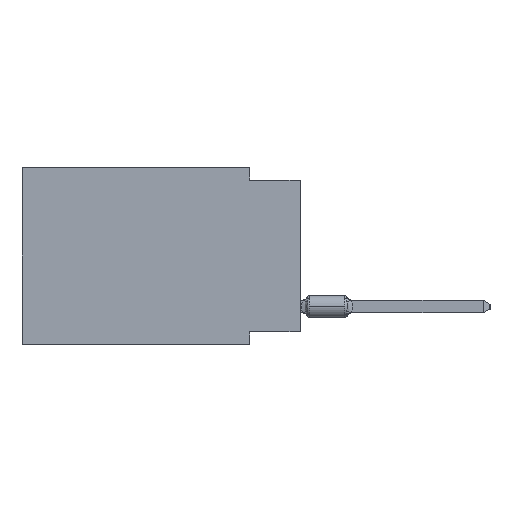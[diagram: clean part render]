
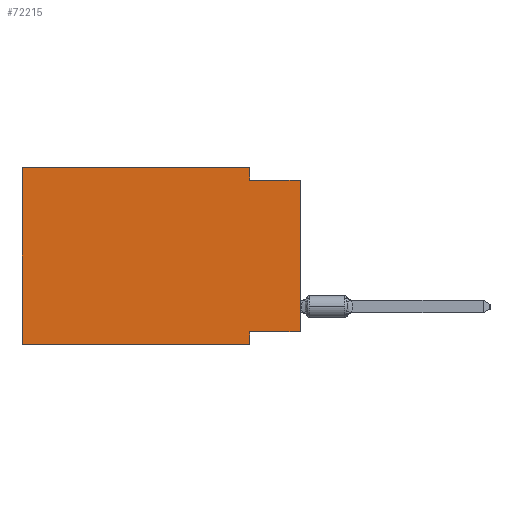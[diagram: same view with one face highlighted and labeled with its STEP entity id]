
A CAD part, left-side view. The second image highlights one B-rep face of the part: STEP entity #72215.
In plain terms, the highlighted planar face has unit normal (-1, 0, 0).
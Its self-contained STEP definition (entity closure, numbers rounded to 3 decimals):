
#387 = VECTOR ( 'NONE', #61756, 1000. ) ;
#1244 = CARTESIAN_POINT ( 'NONE',  ( 0., 13.97, 0. ) ) ;
#3121 = VERTEX_POINT ( 'NONE', #24939 ) ;
#5661 = EDGE_CURVE ( 'NONE', #8910, #59879, #16814, .T. ) ;
#6793 = DIRECTION ( 'NONE',  ( 0., 0., 1. ) ) ;
#7203 = ORIENTED_EDGE ( 'NONE', *, *, #54931, .T. ) ;
#8861 = VERTEX_POINT ( 'NONE', #36413 ) ;
#8910 = VERTEX_POINT ( 'NONE', #65574 ) ;
#9509 = DIRECTION ( 'NONE',  ( 0., 0., -1. ) ) ;
#11728 = DIRECTION ( 'NONE',  ( 0., -1., 0. ) ) ;
#12695 = EDGE_CURVE ( 'NONE', #69014, #20613, #42817, .T. ) ;
#13997 = CARTESIAN_POINT ( 'NONE',  ( 0., 0., -0.635 ) ) ;
#14571 = LINE ( 'NONE', #51498, #34872 ) ;
#16814 = LINE ( 'NONE', #76672, #16905 ) ;
#16905 = VECTOR ( 'NONE', #11728, 1000. ) ;
#17360 = ORIENTED_EDGE ( 'NONE', *, *, #32071, .F. ) ;
#20528 = CARTESIAN_POINT ( 'NONE',  ( 0., 2.54, -0.635 ) ) ;
#20613 = VERTEX_POINT ( 'NONE', #62488 ) ;
#21476 = EDGE_CURVE ( 'NONE', #37753, #20613, #57918, .T. ) ;
#24695 = LINE ( 'NONE', #53091, #24983 ) ;
#24939 = CARTESIAN_POINT ( 'NONE',  ( 0., 2.54, -8.255 ) ) ;
#24983 = VECTOR ( 'NONE', #6793, 1000. ) ;
#25748 = LINE ( 'NONE', #61513, #70456 ) ;
#31001 = AXIS2_PLACEMENT_3D ( 'NONE', #1244, #53358, #31180 ) ;
#31180 = DIRECTION ( 'NONE',  ( 0., 0., -1. ) ) ;
#32071 = EDGE_CURVE ( 'NONE', #40632, #8910, #24695, .T. ) ;
#34872 = VECTOR ( 'NONE', #9509, 1000. ) ;
#36413 = CARTESIAN_POINT ( 'NONE',  ( 0., 2.54, -8.89 ) ) ;
#37660 = LINE ( 'NONE', #61363, #387 ) ;
#37753 = VERTEX_POINT ( 'NONE', #66265 ) ;
#40632 = VERTEX_POINT ( 'NONE', #53017 ) ;
#42088 = FACE_OUTER_BOUND ( 'NONE', #68525, .T. ) ;
#42817 = LINE ( 'NONE', #13997, #49906 ) ;
#42858 = PLANE ( 'NONE',  #31001 ) ;
#44911 = VECTOR ( 'NONE', #75062, 1000. ) ;
#46420 = ORIENTED_EDGE ( 'NONE', *, *, #12695, .F. ) ;
#48350 = ORIENTED_EDGE ( 'NONE', *, *, #75628, .F. ) ;
#48769 = ORIENTED_EDGE ( 'NONE', *, *, #52503, .F. ) ;
#48961 = VECTOR ( 'NONE', #52838, 1000. ) ;
#49906 = VECTOR ( 'NONE', #55627, 1000. ) ;
#51498 = CARTESIAN_POINT ( 'NONE',  ( 0., 2.54, -8.89 ) ) ;
#51747 = LINE ( 'NONE', #58331, #44911 ) ;
#52503 = EDGE_CURVE ( 'NONE', #3121, #8861, #14571, .T. ) ;
#52838 = DIRECTION ( 'NONE',  ( 0., 0., 1. ) ) ;
#53017 = CARTESIAN_POINT ( 'NONE',  ( 0., 13.97, -8.89 ) ) ;
#53091 = CARTESIAN_POINT ( 'NONE',  ( 0., 13.97, 0. ) ) ;
#53358 = DIRECTION ( 'NONE',  ( 1., 0., 0. ) ) ;
#54931 = EDGE_CURVE ( 'NONE', #40632, #8861, #37660, .T. ) ;
#55346 = CARTESIAN_POINT ( 'NONE',  ( 0., 2.54, 0. ) ) ;
#55627 = DIRECTION ( 'NONE',  ( 0., -1., 0. ) ) ;
#57457 = ORIENTED_EDGE ( 'NONE', *, *, #60454, .F. ) ;
#57918 = LINE ( 'NONE', #76163, #48961 ) ;
#58331 = CARTESIAN_POINT ( 'NONE',  ( 0., 0., -8.255 ) ) ;
#59879 = VERTEX_POINT ( 'NONE', #55346 ) ;
#60454 = EDGE_CURVE ( 'NONE', #37753, #3121, #51747, .T. ) ;
#61363 = CARTESIAN_POINT ( 'NONE',  ( 0., 13.97, -8.89 ) ) ;
#61513 = CARTESIAN_POINT ( 'NONE',  ( 0., 2.54, 0. ) ) ;
#61756 = DIRECTION ( 'NONE',  ( 0., -1., 0. ) ) ;
#62488 = CARTESIAN_POINT ( 'NONE',  ( 0., 0., -0.635 ) ) ;
#65574 = CARTESIAN_POINT ( 'NONE',  ( 0., 13.97, 0. ) ) ;
#66265 = CARTESIAN_POINT ( 'NONE',  ( 0., 0., -8.255 ) ) ;
#68525 = EDGE_LOOP ( 'NONE', ( #74449, #46420, #48350, #74242, #17360, #7203, #48769, #57457 ) ) ;
#69014 = VERTEX_POINT ( 'NONE', #20528 ) ;
#70456 = VECTOR ( 'NONE', #72404, 1000. ) ;
#72215 = ADVANCED_FACE ( 'NONE', ( #42088 ), #42858, .F. ) ;
#72404 = DIRECTION ( 'NONE',  ( 0., 0., -1. ) ) ;
#74242 = ORIENTED_EDGE ( 'NONE', *, *, #5661, .F. ) ;
#74449 = ORIENTED_EDGE ( 'NONE', *, *, #21476, .T. ) ;
#75062 = DIRECTION ( 'NONE',  ( 0., 1., 0. ) ) ;
#75628 = EDGE_CURVE ( 'NONE', #59879, #69014, #25748, .T. ) ;
#76163 = CARTESIAN_POINT ( 'NONE',  ( 0., 0., 0. ) ) ;
#76672 = CARTESIAN_POINT ( 'NONE',  ( 0., 13.97, 0. ) ) ;
